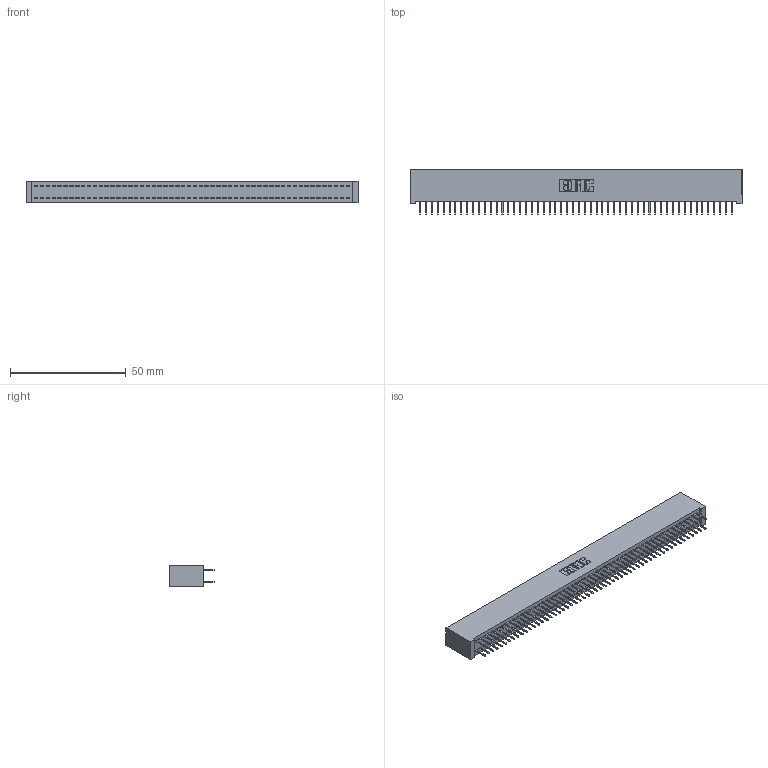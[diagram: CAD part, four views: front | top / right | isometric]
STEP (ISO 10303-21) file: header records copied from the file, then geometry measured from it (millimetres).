
FILE_DESCRIPTION (( 'STEP AP203' ), '1' );
FILE_NAME ('342-108-524-201.STEP', '2018-08-14T07:41:25', ( '' ), ( '' ), 'SwSTEP 2.0', 'SolidWorks 2016', '' );
FILE_SCHEMA (( 'CONFIG_CONTROL_DESIGN' ));
Length unit declared in the file: inch
Products named in the file (3): 342 Part_Lugless; 345-292-001_345-293-124; 342-108-524-201
Assembly tree (109 placements, depth 2):
  342-108-524-201
    342 Part_Lugless
    345-292-001_345-293-124  x108
Bounding box: 143.41 x 19.69 x 9.4 mm (x, y, z)
Volume: 13218.1 mm3; surface area: 21832.5 mm2
Topology: 109 solids, 109 shells, 6150 faces, 17447 edges, 11198 vertices
Faces by surface type: plane 4598, cylinder 1552
Entity records: 32853 total; most frequent: CARTESIAN_POINT 5426, ORIENTED_EDGE 5362, DIRECTION 4609, EDGE_CURVE 2681, VECTOR 2565, LINE 2565, VERTEX_POINT 1782, AXIS2_PLACEMENT_3D 1022
